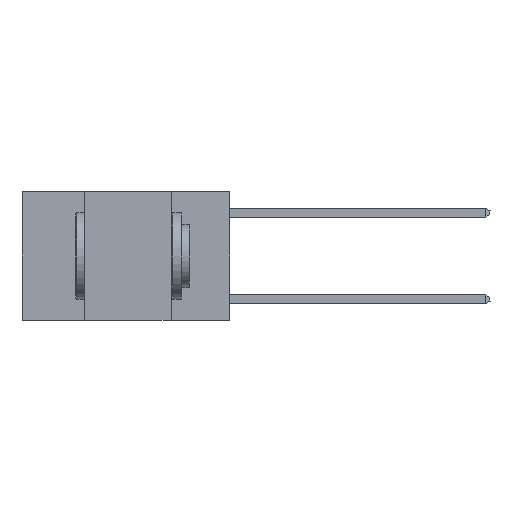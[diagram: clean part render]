
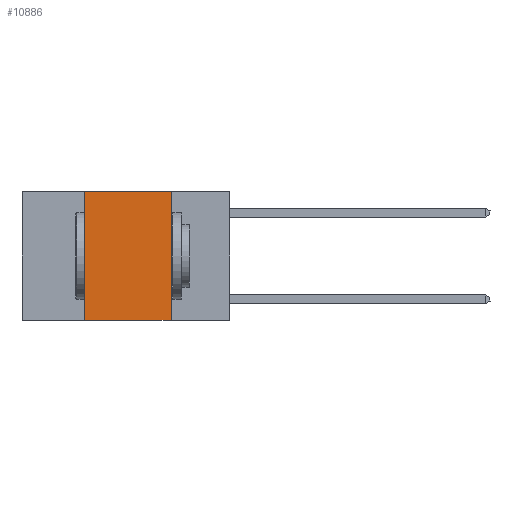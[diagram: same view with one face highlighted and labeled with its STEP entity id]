
A CAD part, left-side view. The second image highlights one B-rep face of the part: STEP entity #10886.
In plain terms, the highlighted planar face has unit normal (-1, 0, 0).
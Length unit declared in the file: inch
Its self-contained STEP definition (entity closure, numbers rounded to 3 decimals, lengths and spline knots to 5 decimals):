
#166 = AXIS2_PLACEMENT_3D ( 'NONE', #19668, #6526, #18121 ) ;
#769 = LINE ( 'NONE', #10728, #18001 ) ;
#1411 = PLANE ( 'NONE',  #166 ) ;
#3123 = EDGE_LOOP ( 'NONE', ( #11161, #13001, #15430, #20233 ) ) ;
#3520 = VECTOR ( 'NONE', #19301, 39.37008 ) ;
#4551 = CARTESIAN_POINT ( 'NONE',  ( 0., 0.17, -0.37 ) ) ;
#4821 = VERTEX_POINT ( 'NONE', #8745 ) ;
#6526 = DIRECTION ( 'NONE',  ( 1., 0., 0. ) ) ;
#6823 = EDGE_CURVE ( 'NONE', #4821, #8047, #11028, .T. ) ;
#6853 = LINE ( 'NONE', #16573, #19518 ) ;
#8026 = LINE ( 'NONE', #11088, #3520 ) ;
#8047 = VERTEX_POINT ( 'NONE', #4551 ) ;
#8745 = CARTESIAN_POINT ( 'NONE',  ( 0., 0.42, -0.37 ) ) ;
#8965 = DIRECTION ( 'NONE',  ( 0., 0., 1. ) ) ;
#9017 = VERTEX_POINT ( 'NONE', #15062 ) ;
#10728 = CARTESIAN_POINT ( 'NONE',  ( 0., 0.42, 0. ) ) ;
#10886 = ADVANCED_FACE ( 'NONE', ( #18595 ), #1411, .F. ) ;
#11028 = LINE ( 'NONE', #18196, #18768 ) ;
#11088 = CARTESIAN_POINT ( 'NONE',  ( 0., 0.17, 0. ) ) ;
#11161 = ORIENTED_EDGE ( 'NONE', *, *, #16837, .F. ) ;
#11719 = CARTESIAN_POINT ( 'NONE',  ( 0., 0.17, 0. ) ) ;
#13001 = ORIENTED_EDGE ( 'NONE', *, *, #17759, .F. ) ;
#13532 = EDGE_CURVE ( 'NONE', #4821, #9017, #769, .T. ) ;
#15062 = CARTESIAN_POINT ( 'NONE',  ( 0., 0.42, 0. ) ) ;
#15218 = VERTEX_POINT ( 'NONE', #11719 ) ;
#15430 = ORIENTED_EDGE ( 'NONE', *, *, #13532, .F. ) ;
#16573 = CARTESIAN_POINT ( 'NONE',  ( 0., 0.6, 0. ) ) ;
#16837 = EDGE_CURVE ( 'NONE', #15218, #8047, #8026, .T. ) ;
#17759 = EDGE_CURVE ( 'NONE', #9017, #15218, #6853, .T. ) ;
#18001 = VECTOR ( 'NONE', #8965, 39.37008 ) ;
#18121 = DIRECTION ( 'NONE',  ( 0., 0., -1. ) ) ;
#18196 = CARTESIAN_POINT ( 'NONE',  ( 0., 0.6, -0.37 ) ) ;
#18595 = FACE_OUTER_BOUND ( 'NONE', #3123, .T. ) ;
#18768 = VECTOR ( 'NONE', #19808, 39.37008 ) ;
#19301 = DIRECTION ( 'NONE',  ( 0., 0., -1. ) ) ;
#19518 = VECTOR ( 'NONE', #19877, 39.37008 ) ;
#19668 = CARTESIAN_POINT ( 'NONE',  ( 0., 0.6, 0. ) ) ;
#19808 = DIRECTION ( 'NONE',  ( 0., -1., 0. ) ) ;
#19877 = DIRECTION ( 'NONE',  ( 0., -1., 0. ) ) ;
#20233 = ORIENTED_EDGE ( 'NONE', *, *, #6823, .T. ) ;
